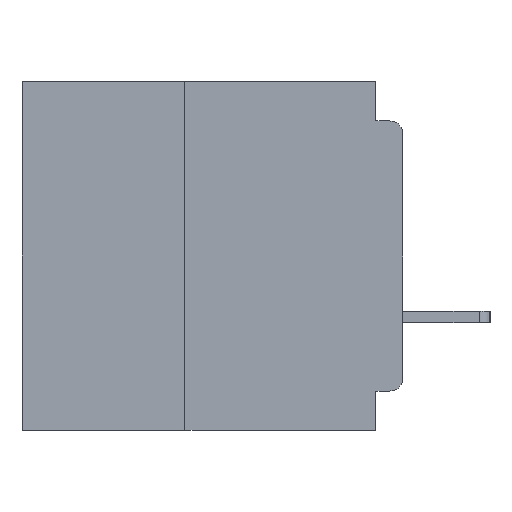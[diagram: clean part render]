
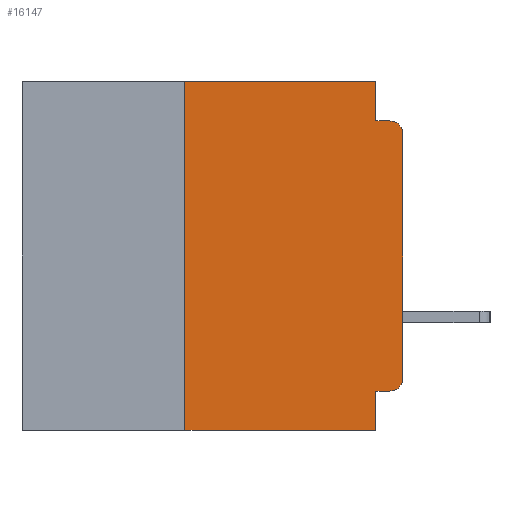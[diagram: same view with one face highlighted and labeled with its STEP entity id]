
A CAD part, left-side view. The second image highlights one B-rep face of the part: STEP entity #16147.
In plain terms, the highlighted planar face has unit normal (-1, 0, 0).
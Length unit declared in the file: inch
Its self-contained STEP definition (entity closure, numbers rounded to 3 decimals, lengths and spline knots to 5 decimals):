
#188 = AXIS2_PLACEMENT_3D ( 'NONE', #35623, #35514, #35204 ) ;
#633 = DIRECTION ( 'NONE',  ( 0., 1., 0. ) ) ;
#737 = LINE ( 'NONE', #14656, #18390 ) ;
#1128 = FACE_OUTER_BOUND ( 'NONE', #10484, .T. ) ;
#1348 = CARTESIAN_POINT ( 'NONE',  ( 0., 0.015, -0.34 ) ) ;
#1615 = EDGE_CURVE ( 'NONE', #34115, #43744, #38780, .T. ) ;
#1946 = EDGE_CURVE ( 'NONE', #8201, #2483, #44166, .T. ) ;
#2483 = VERTEX_POINT ( 'NONE', #28242 ) ;
#2870 = EDGE_CURVE ( 'NONE', #2483, #26746, #15238, .T. ) ;
#3327 = VECTOR ( 'NONE', #28159, 39.37008 ) ;
#3451 = VECTOR ( 'NONE', #45295, 39.37008 ) ;
#4697 = CARTESIAN_POINT ( 'NONE',  ( 0., 0.25, -0.4 ) ) ;
#4947 = DIRECTION ( 'NONE',  ( 0., 0., -1. ) ) ;
#5097 = CARTESIAN_POINT ( 'NONE',  ( 0., 0.437, 0. ) ) ;
#6404 = EDGE_CURVE ( 'NONE', #15431, #43744, #30362, .T. ) ;
#7590 = CARTESIAN_POINT ( 'NONE',  ( 0., 0.031, -0.4 ) ) ;
#8201 = VERTEX_POINT ( 'NONE', #21347 ) ;
#8779 = EDGE_CURVE ( 'NONE', #15431, #36402, #737, .T. ) ;
#8804 = PLANE ( 'NONE',  #45114 ) ;
#9565 = DIRECTION ( 'NONE',  ( 0., -1., 0. ) ) ;
#10021 = EDGE_CURVE ( 'NONE', #42837, #34115, #31006, .T. ) ;
#10484 = EDGE_LOOP ( 'NONE', ( #39310, #39871, #24386, #32206, #32749, #33328, #12491, #24068, #36827, #21982 ) ) ;
#10609 = AXIS2_PLACEMENT_3D ( 'NONE', #1348, #26050, #4947 ) ;
#10886 = LINE ( 'NONE', #23303, #28543 ) ;
#12329 = DIRECTION ( 'NONE',  ( 0., 0., -1. ) ) ;
#12491 = ORIENTED_EDGE ( 'NONE', *, *, #6404, .T. ) ;
#13357 = CARTESIAN_POINT ( 'NONE',  ( 0., 0.25, 0. ) ) ;
#13500 = EDGE_CURVE ( 'NONE', #40774, #38658, #23448, .T. ) ;
#14173 = CARTESIAN_POINT ( 'NONE',  ( 0., 0.031, -0.355 ) ) ;
#14656 = CARTESIAN_POINT ( 'NONE',  ( 0., 0.25, -0.4 ) ) ;
#15238 = CIRCLE ( 'NONE', #188, 0.015 ) ;
#15431 = VERTEX_POINT ( 'NONE', #4697 ) ;
#16147 = ADVANCED_FACE ( 'NONE', ( #1128 ), #8804, .F. ) ;
#16300 = CARTESIAN_POINT ( 'NONE',  ( 0., 0.031, 0. ) ) ;
#17635 = CARTESIAN_POINT ( 'NONE',  ( 0., 0.437, -0.4 ) ) ;
#18390 = VECTOR ( 'NONE', #35983, 39.37008 ) ;
#20133 = EDGE_CURVE ( 'NONE', #36402, #40774, #10886, .T. ) ;
#21347 = CARTESIAN_POINT ( 'NONE',  ( 0., 0., -0.34 ) ) ;
#21584 = VECTOR ( 'NONE', #633, 39.37008 ) ;
#21982 = ORIENTED_EDGE ( 'NONE', *, *, #43904, .T. ) ;
#23303 = CARTESIAN_POINT ( 'NONE',  ( 0., 0.437, 0. ) ) ;
#23448 = LINE ( 'NONE', #16300, #32877 ) ;
#23496 = CARTESIAN_POINT ( 'NONE',  ( 0., 0.015, -0.355 ) ) ;
#24068 = ORIENTED_EDGE ( 'NONE', *, *, #1615, .F. ) ;
#24333 = VECTOR ( 'NONE', #33830, 39.37008 ) ;
#24386 = ORIENTED_EDGE ( 'NONE', *, *, #26505, .F. ) ;
#24861 = VECTOR ( 'NONE', #9565, 39.37008 ) ;
#26050 = DIRECTION ( 'NONE',  ( -1., 0., 0. ) ) ;
#26505 = EDGE_CURVE ( 'NONE', #38658, #26746, #42499, .T. ) ;
#26746 = VERTEX_POINT ( 'NONE', #42652 ) ;
#26866 = DIRECTION ( 'NONE',  ( 0., -1., 0. ) ) ;
#27046 = CIRCLE ( 'NONE', #10609, 0.015 ) ;
#27106 = CARTESIAN_POINT ( 'NONE',  ( 0., 0., -0.045 ) ) ;
#28159 = DIRECTION ( 'NONE',  ( 0., -1., 0. ) ) ;
#28242 = CARTESIAN_POINT ( 'NONE',  ( 0., 0., -0.06 ) ) ;
#28543 = VECTOR ( 'NONE', #26866, 39.37008 ) ;
#28905 = CARTESIAN_POINT ( 'NONE',  ( 0., 0., -0.355 ) ) ;
#30362 = LINE ( 'NONE', #17635, #3327 ) ;
#31006 = LINE ( 'NONE', #28905, #21584 ) ;
#32206 = ORIENTED_EDGE ( 'NONE', *, *, #13500, .F. ) ;
#32749 = ORIENTED_EDGE ( 'NONE', *, *, #20133, .F. ) ;
#32877 = VECTOR ( 'NONE', #40966, 39.37008 ) ;
#33328 = ORIENTED_EDGE ( 'NONE', *, *, #8779, .F. ) ;
#33482 = DIRECTION ( 'NONE',  ( 1., 0., 0. ) ) ;
#33662 = CARTESIAN_POINT ( 'NONE',  ( 0., 0., 0. ) ) ;
#33830 = DIRECTION ( 'NONE',  ( 0., 0., 1. ) ) ;
#34115 = VERTEX_POINT ( 'NONE', #14173 ) ;
#35204 = DIRECTION ( 'NONE',  ( 0., 0., -1. ) ) ;
#35514 = DIRECTION ( 'NONE',  ( -1., 0., 0. ) ) ;
#35623 = CARTESIAN_POINT ( 'NONE',  ( 0., 0.015, -0.06 ) ) ;
#35983 = DIRECTION ( 'NONE',  ( 0., 0., 1. ) ) ;
#36402 = VERTEX_POINT ( 'NONE', #13357 ) ;
#36827 = ORIENTED_EDGE ( 'NONE', *, *, #10021, .F. ) ;
#38658 = VERTEX_POINT ( 'NONE', #40619 ) ;
#38780 = LINE ( 'NONE', #45237, #3451 ) ;
#39310 = ORIENTED_EDGE ( 'NONE', *, *, #1946, .T. ) ;
#39871 = ORIENTED_EDGE ( 'NONE', *, *, #2870, .T. ) ;
#40619 = CARTESIAN_POINT ( 'NONE',  ( 0., 0.031, -0.045 ) ) ;
#40688 = CARTESIAN_POINT ( 'NONE',  ( 0., 0.031, 0. ) ) ;
#40774 = VERTEX_POINT ( 'NONE', #40688 ) ;
#40966 = DIRECTION ( 'NONE',  ( 0., 0., -1. ) ) ;
#42499 = LINE ( 'NONE', #27106, #24861 ) ;
#42652 = CARTESIAN_POINT ( 'NONE',  ( 0., 0.015, -0.045 ) ) ;
#42837 = VERTEX_POINT ( 'NONE', #23496 ) ;
#43744 = VERTEX_POINT ( 'NONE', #7590 ) ;
#43904 = EDGE_CURVE ( 'NONE', #42837, #8201, #27046, .T. ) ;
#44166 = LINE ( 'NONE', #33662, #24333 ) ;
#45114 = AXIS2_PLACEMENT_3D ( 'NONE', #5097, #33482, #12329 ) ;
#45237 = CARTESIAN_POINT ( 'NONE',  ( 0., 0.031, -0.4 ) ) ;
#45295 = DIRECTION ( 'NONE',  ( 0., 0., -1. ) ) ;
